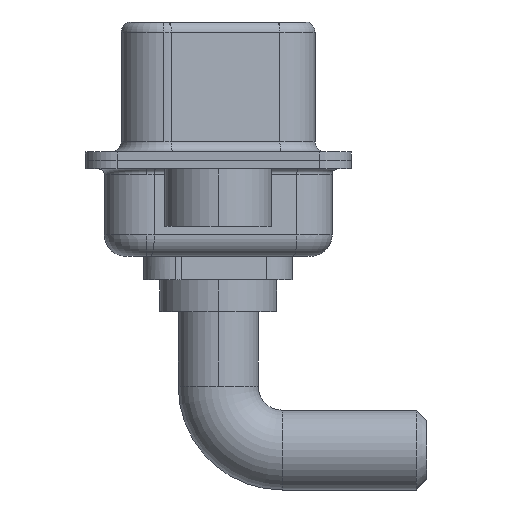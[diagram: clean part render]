
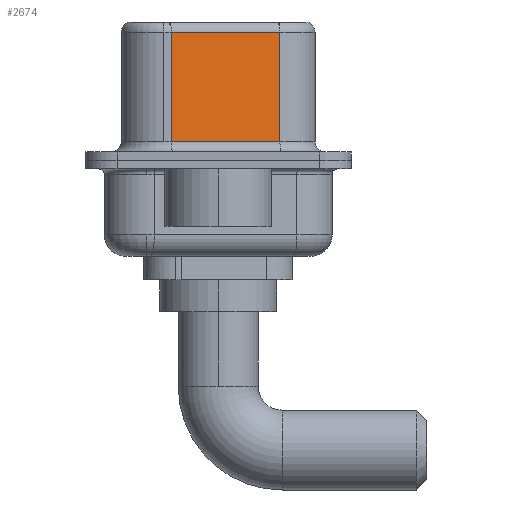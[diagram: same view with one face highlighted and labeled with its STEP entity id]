
A CAD part, left-side view. The second image highlights one B-rep face of the part: STEP entity #2674.
In plain terms, the highlighted planar face has unit normal (-0.985, -0.174, 0).
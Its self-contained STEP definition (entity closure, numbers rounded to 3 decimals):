
#8 = ORIENTED_EDGE ( 'NONE', *, *, #12639, .T. ) ;
#338 = LINE ( 'NONE', #11838, #6816 ) ;
#1625 = EDGE_CURVE ( 'NONE', #14941, #12062, #12968, .T. ) ;
#1641 = DIRECTION ( 'NONE',  ( 0.174, -0.985, 0. ) ) ;
#2023 = AXIS2_PLACEMENT_3D ( 'NONE', #8063, #9284, #13721 ) ;
#2674 = ADVANCED_FACE ( 'NONE', ( #11823 ), #3084, .F. ) ;
#2790 = CARTESIAN_POINT ( 'NONE',  ( 4.58, -2.897, 0.9 ) ) ;
#3084 = PLANE ( 'NONE',  #2023 ) ;
#3471 = EDGE_LOOP ( 'NONE', ( #8169, #8, #6643, #4505 ) ) ;
#4379 = LINE ( 'NONE', #7985, #7124 ) ;
#4505 = ORIENTED_EDGE ( 'NONE', *, *, #1625, .T. ) ;
#5210 = CARTESIAN_POINT ( 'NONE',  ( 4.58, -2.897, 0.9 ) ) ;
#5997 = VERTEX_POINT ( 'NONE', #14505 ) ;
#6643 = ORIENTED_EDGE ( 'NONE', *, *, #10813, .T. ) ;
#6652 = CARTESIAN_POINT ( 'NONE',  ( 3.68, 2.203, 6.02 ) ) ;
#6816 = VECTOR ( 'NONE', #8985, 1000. ) ;
#7124 = VECTOR ( 'NONE', #14263, 1000. ) ;
#7441 = VECTOR ( 'NONE', #1641, 1000. ) ;
#7985 = CARTESIAN_POINT ( 'NONE',  ( 4.58, -2.897, 6.02 ) ) ;
#8063 = CARTESIAN_POINT ( 'NONE',  ( 4.58, -2.897, 6.52 ) ) ;
#8169 = ORIENTED_EDGE ( 'NONE', *, *, #10597, .F. ) ;
#8337 = DIRECTION ( 'NONE',  ( 0., 0., -1. ) ) ;
#8985 = DIRECTION ( 'NONE',  ( 0., 0., -1. ) ) ;
#9217 = CARTESIAN_POINT ( 'NONE',  ( 3.68, 2.203, 0.9 ) ) ;
#9284 = DIRECTION ( 'NONE',  ( 0.985, 0.174, 0. ) ) ;
#9874 = VERTEX_POINT ( 'NONE', #6652 ) ;
#10597 = EDGE_CURVE ( 'NONE', #5997, #12062, #12258, .T. ) ;
#10723 = VECTOR ( 'NONE', #8337, 1000. ) ;
#10813 = EDGE_CURVE ( 'NONE', #9874, #14941, #338, .T. ) ;
#11823 = FACE_OUTER_BOUND ( 'NONE', #3471, .T. ) ;
#11838 = CARTESIAN_POINT ( 'NONE',  ( 3.68, 2.203, 6.52 ) ) ;
#12062 = VERTEX_POINT ( 'NONE', #2790 ) ;
#12258 = LINE ( 'NONE', #13302, #10723 ) ;
#12639 = EDGE_CURVE ( 'NONE', #5997, #9874, #4379, .T. ) ;
#12968 = LINE ( 'NONE', #5210, #7441 ) ;
#13302 = CARTESIAN_POINT ( 'NONE',  ( 4.58, -2.897, 6.52 ) ) ;
#13721 = DIRECTION ( 'NONE',  ( -0.174, 0.985, 0. ) ) ;
#14263 = DIRECTION ( 'NONE',  ( -0.174, 0.985, 0. ) ) ;
#14505 = CARTESIAN_POINT ( 'NONE',  ( 4.58, -2.897, 6.02 ) ) ;
#14941 = VERTEX_POINT ( 'NONE', #9217 ) ;
